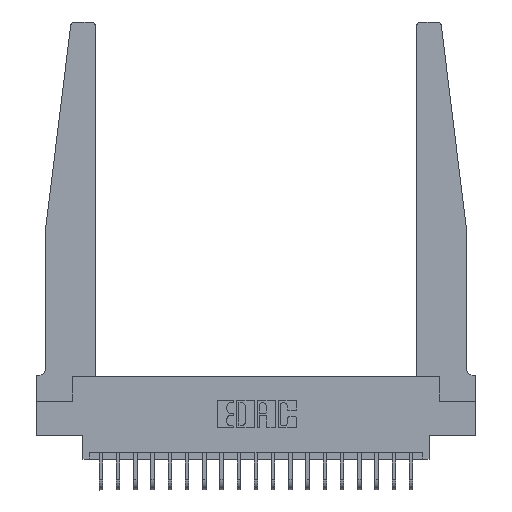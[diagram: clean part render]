
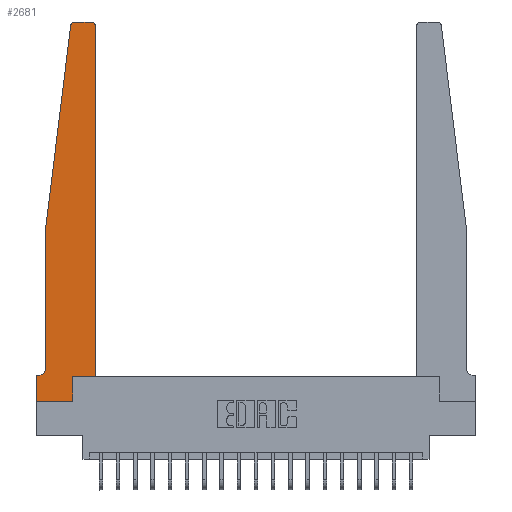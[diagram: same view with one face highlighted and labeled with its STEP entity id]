
A CAD part, top view. The second image highlights one B-rep face of the part: STEP entity #2681.
In plain terms, the highlighted planar face has unit normal (0, 0, 1).
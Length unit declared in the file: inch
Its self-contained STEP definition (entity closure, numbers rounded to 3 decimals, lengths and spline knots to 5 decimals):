
#35 = CARTESIAN_POINT ( 'NONE',  ( 0.25, 2.75, 0.37 ) ) ;
#265 = CIRCLE ( 'NONE', #17938, 0.03 ) ;
#1347 = VECTOR ( 'NONE', #19391, 39.37008 ) ;
#1453 = EDGE_CURVE ( 'NONE', #4234, #19075, #265, .T. ) ;
#1914 = VERTEX_POINT ( 'NONE', #6975 ) ;
#2021 = ORIENTED_EDGE ( 'NONE', *, *, #10067, .T. ) ;
#2093 = ORIENTED_EDGE ( 'NONE', *, *, #16156, .T. ) ;
#2445 = DIRECTION ( 'NONE',  ( 0., 0., 1. ) ) ;
#2681 = ADVANCED_FACE ( 'NONE', ( #17692 ), #5054, .T. ) ;
#3121 = ORIENTED_EDGE ( 'NONE', *, *, #11770, .T. ) ;
#3269 = CARTESIAN_POINT ( 'NONE',  ( 0.27653, 2.75, 0.37 ) ) ;
#3286 = EDGE_CURVE ( 'NONE', #21007, #20118, #8939, .T. ) ;
#3368 = EDGE_CURVE ( 'NONE', #16637, #4234, #5406, .T. ) ;
#3874 = DIRECTION ( 'NONE',  ( 0., 1., 0. ) ) ;
#3926 = LINE ( 'NONE', #9689, #17869 ) ;
#3965 = DIRECTION ( 'NONE',  ( 0., 0., -1. ) ) ;
#4154 = DIRECTION ( 'NONE',  ( 0., -1., 0. ) ) ;
#4174 = CARTESIAN_POINT ( 'NONE',  ( 0., 0., 0.37 ) ) ;
#4234 = VERTEX_POINT ( 'NONE', #3269 ) ;
#5054 = PLANE ( 'NONE',  #19702 ) ;
#5275 = CARTESIAN_POINT ( 'NONE',  ( 0., 0.1875, 0.37 ) ) ;
#5286 = ORIENTED_EDGE ( 'NONE', *, *, #19551, .T. ) ;
#5406 = LINE ( 'NONE', #35, #13980 ) ;
#5489 = ORIENTED_EDGE ( 'NONE', *, *, #3368, .T. ) ;
#5853 = CARTESIAN_POINT ( 'NONE',  ( 0.065, 1.25, 0.37 ) ) ;
#5968 = VECTOR ( 'NONE', #20546, 39.37008 ) ;
#6001 = VECTOR ( 'NONE', #3874, 39.37008 ) ;
#6030 = CARTESIAN_POINT ( 'NONE',  ( 0.24675, 2.72367, 0.37 ) ) ;
#6376 = VECTOR ( 'NONE', #18529, 39.37008 ) ;
#6659 = VERTEX_POINT ( 'NONE', #4174 ) ;
#6975 = CARTESIAN_POINT ( 'NONE',  ( 0.065, 1.25, 0.37 ) ) ;
#7077 = CARTESIAN_POINT ( 'NONE',  ( 0.065, 0.2375, 0.37 ) ) ;
#7179 = CARTESIAN_POINT ( 'NONE',  ( 0.2605, 0.18, 0.37 ) ) ;
#7221 = VERTEX_POINT ( 'NONE', #17439 ) ;
#7581 = LINE ( 'NONE', #16165, #7844 ) ;
#7659 = CARTESIAN_POINT ( 'NONE',  ( 0.015, 0.2375, 0.37 ) ) ;
#7737 = VERTEX_POINT ( 'NONE', #10435 ) ;
#7844 = VECTOR ( 'NONE', #4154, 39.37008 ) ;
#8053 = EDGE_CURVE ( 'NONE', #8054, #21007, #3926, .T. ) ;
#8054 = VERTEX_POINT ( 'NONE', #18287 ) ;
#8154 = AXIS2_PLACEMENT_3D ( 'NONE', #19721, #2445, #12901 ) ;
#8232 = DIRECTION ( 'NONE',  ( -1., 0., 0. ) ) ;
#8347 = CARTESIAN_POINT ( 'NONE',  ( 0.425, 0.18, 0.37 ) ) ;
#8443 = CARTESIAN_POINT ( 'NONE',  ( 0.065, 1.25, 0.37 ) ) ;
#8939 = LINE ( 'NONE', #8941, #6001 ) ;
#8941 = CARTESIAN_POINT ( 'NONE',  ( 0.425, 0.18, 0.37 ) ) ;
#9046 = CARTESIAN_POINT ( 'NONE',  ( 0.27653, 2.72, 0.37 ) ) ;
#9689 = CARTESIAN_POINT ( 'NONE',  ( 0.425, 0.18, 0.37 ) ) ;
#9847 = ORIENTED_EDGE ( 'NONE', *, *, #14806, .T. ) ;
#10067 = EDGE_CURVE ( 'NONE', #11343, #7737, #21516, .T. ) ;
#10435 = CARTESIAN_POINT ( 'NONE',  ( 0., 0.1875, 0.37 ) ) ;
#10491 = DIRECTION ( 'NONE',  ( -1., 0., 0. ) ) ;
#10764 = DIRECTION ( 'NONE',  ( 1., 0., 0. ) ) ;
#11343 = VERTEX_POINT ( 'NONE', #18363 ) ;
#11367 = ORIENTED_EDGE ( 'NONE', *, *, #17698, .T. ) ;
#11600 = LINE ( 'NONE', #19132, #21765 ) ;
#11770 = EDGE_CURVE ( 'NONE', #6659, #7221, #11600, .T. ) ;
#11857 = EDGE_CURVE ( 'NONE', #7221, #8054, #17230, .T. ) ;
#12239 = ORIENTED_EDGE ( 'NONE', *, *, #20149, .T. ) ;
#12331 = ORIENTED_EDGE ( 'NONE', *, *, #8053, .T. ) ;
#12529 = DIRECTION ( 'NONE',  ( 0., 0., 1. ) ) ;
#12901 = DIRECTION ( 'NONE',  ( 1., 0., 0. ) ) ;
#13485 = VERTEX_POINT ( 'NONE', #7077 ) ;
#13980 = VECTOR ( 'NONE', #10491, 39.37008 ) ;
#14500 = LINE ( 'NONE', #5853, #1347 ) ;
#14806 = EDGE_CURVE ( 'NONE', #1914, #13485, #21893, .T. ) ;
#15114 = CARTESIAN_POINT ( 'NONE',  ( 0.065, 0.1875, 0.37 ) ) ;
#16156 = EDGE_CURVE ( 'NONE', #20118, #16637, #16538, .T. ) ;
#16165 = CARTESIAN_POINT ( 'NONE',  ( 0., 0., 0.37 ) ) ;
#16353 = AXIS2_PLACEMENT_3D ( 'NONE', #7659, #3965, #19630 ) ;
#16538 = CIRCLE ( 'NONE', #8154, 0.03 ) ;
#16637 = VERTEX_POINT ( 'NONE', #17103 ) ;
#16742 = ORIENTED_EDGE ( 'NONE', *, *, #3286, .T. ) ;
#17103 = CARTESIAN_POINT ( 'NONE',  ( 0.395, 2.75, 0.37 ) ) ;
#17230 = LINE ( 'NONE', #7179, #5968 ) ;
#17272 = DIRECTION ( 'NONE',  ( 0., 0., 1. ) ) ;
#17439 = CARTESIAN_POINT ( 'NONE',  ( 0.2605, 0., 0.37 ) ) ;
#17692 = FACE_OUTER_BOUND ( 'NONE', #21644, .T. ) ;
#17698 = EDGE_CURVE ( 'NONE', #13485, #11343, #20737, .T. ) ;
#17869 = VECTOR ( 'NONE', #21626, 39.37008 ) ;
#17938 = AXIS2_PLACEMENT_3D ( 'NONE', #9046, #12529, #10764 ) ;
#18287 = CARTESIAN_POINT ( 'NONE',  ( 0.2605, 0.18, 0.37 ) ) ;
#18363 = CARTESIAN_POINT ( 'NONE',  ( 0.015, 0.1875, 0.37 ) ) ;
#18529 = DIRECTION ( 'NONE',  ( 0., -1., 0. ) ) ;
#19069 = ORIENTED_EDGE ( 'NONE', *, *, #1453, .T. ) ;
#19075 = VERTEX_POINT ( 'NONE', #6030 ) ;
#19132 = CARTESIAN_POINT ( 'NONE',  ( 0., 0., 0.37 ) ) ;
#19391 = DIRECTION ( 'NONE',  ( -0.122, -0.992, 0. ) ) ;
#19551 = EDGE_CURVE ( 'NONE', #19075, #1914, #14500, .T. ) ;
#19630 = DIRECTION ( 'NONE',  ( -1., 0., 0. ) ) ;
#19702 = AXIS2_PLACEMENT_3D ( 'NONE', #5275, #17272, #20547 ) ;
#19721 = CARTESIAN_POINT ( 'NONE',  ( 0.395, 2.72, 0.37 ) ) ;
#19926 = VECTOR ( 'NONE', #8232, 39.37008 ) ;
#20118 = VERTEX_POINT ( 'NONE', #20783 ) ;
#20149 = EDGE_CURVE ( 'NONE', #7737, #6659, #7581, .T. ) ;
#20546 = DIRECTION ( 'NONE',  ( 0., 1., 0. ) ) ;
#20547 = DIRECTION ( 'NONE',  ( 1., 0., 0. ) ) ;
#20571 = ORIENTED_EDGE ( 'NONE', *, *, #11857, .T. ) ;
#20698 = DIRECTION ( 'NONE',  ( 1., 0., 0. ) ) ;
#20737 = CIRCLE ( 'NONE', #16353, 0.05 ) ;
#20783 = CARTESIAN_POINT ( 'NONE',  ( 0.425, 2.72, 0.37 ) ) ;
#21007 = VERTEX_POINT ( 'NONE', #8347 ) ;
#21516 = LINE ( 'NONE', #15114, #19926 ) ;
#21626 = DIRECTION ( 'NONE',  ( 1., 0., 0. ) ) ;
#21644 = EDGE_LOOP ( 'NONE', ( #5489, #19069, #5286, #9847, #11367, #2021, #12239, #3121, #20571, #12331, #16742, #2093 ) ) ;
#21765 = VECTOR ( 'NONE', #20698, 39.37008 ) ;
#21893 = LINE ( 'NONE', #8443, #6376 ) ;
